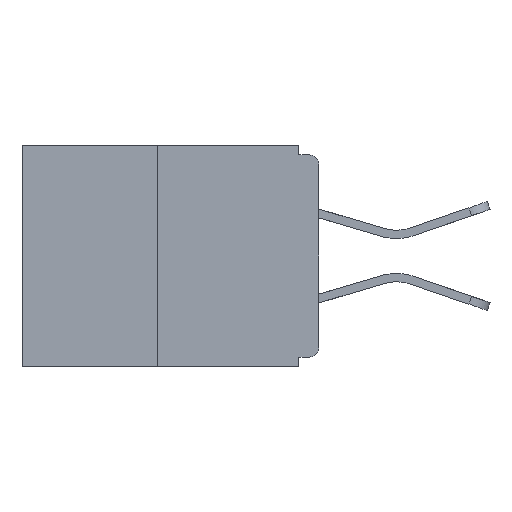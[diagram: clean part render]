
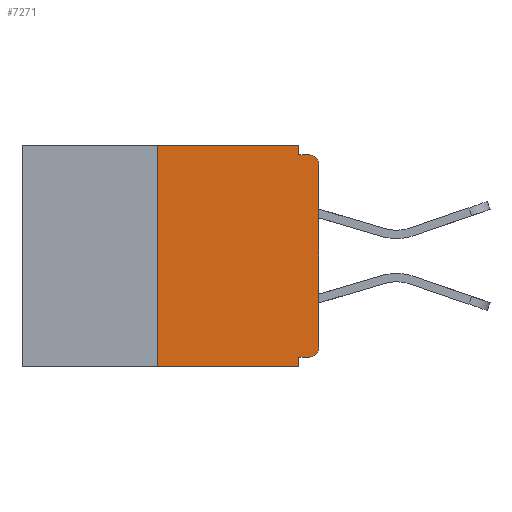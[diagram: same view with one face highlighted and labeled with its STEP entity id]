
A CAD part, left-side view. The second image highlights one B-rep face of the part: STEP entity #7271.
In plain terms, the highlighted planar face has unit normal (-1, 0, 0).
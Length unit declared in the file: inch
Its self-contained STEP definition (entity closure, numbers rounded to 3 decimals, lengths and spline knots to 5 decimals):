
#245 = VECTOR ( 'NONE', #8367, 39.37008 ) ;
#372 = ORIENTED_EDGE ( 'NONE', *, *, #16905, .F. ) ;
#413 = CARTESIAN_POINT ( 'NONE',  ( 0., 0.015, -0.328 ) ) ;
#485 = VECTOR ( 'NONE', #21618, 39.37008 ) ;
#593 = EDGE_CURVE ( 'NONE', #3651, #3572, #9509, .T. ) ;
#948 = EDGE_CURVE ( 'NONE', #8025, #3651, #18871, .T. ) ;
#999 = DIRECTION ( 'NONE',  ( -1., 0., 0. ) ) ;
#1178 = VERTEX_POINT ( 'NONE', #14687 ) ;
#1480 = CARTESIAN_POINT ( 'NONE',  ( 0., 0.25, 0. ) ) ;
#1798 = CARTESIAN_POINT ( 'NONE',  ( 0., 0.031, -0.343 ) ) ;
#1896 = DIRECTION ( 'NONE',  ( 0., 0., -1. ) ) ;
#2040 = CARTESIAN_POINT ( 'NONE',  ( 0., 0.25, -0.343 ) ) ;
#2289 = VECTOR ( 'NONE', #14807, 39.37008 ) ;
#2861 = VERTEX_POINT ( 'NONE', #12835 ) ;
#3013 = VERTEX_POINT ( 'NONE', #2040 ) ;
#3572 = VERTEX_POINT ( 'NONE', #19977 ) ;
#3651 = VERTEX_POINT ( 'NONE', #19838 ) ;
#4171 = DIRECTION ( 'NONE',  ( -1., 0., 0. ) ) ;
#4330 = VERTEX_POINT ( 'NONE', #413 ) ;
#4345 = VECTOR ( 'NONE', #11324, 39.37008 ) ;
#4585 = VERTEX_POINT ( 'NONE', #1798 ) ;
#5065 = CARTESIAN_POINT ( 'NONE',  ( 0., 0.015, -0.015 ) ) ;
#5356 = ORIENTED_EDGE ( 'NONE', *, *, #21210, .T. ) ;
#5528 = CARTESIAN_POINT ( 'NONE',  ( 0., 0.25, 0. ) ) ;
#5738 = CARTESIAN_POINT ( 'NONE',  ( 0., 0.46, -0.343 ) ) ;
#6963 = LINE ( 'NONE', #22767, #2289 ) ;
#7044 = ORIENTED_EDGE ( 'NONE', *, *, #593, .F. ) ;
#7089 = CARTESIAN_POINT ( 'NONE',  ( 0., 0., -0.015 ) ) ;
#7271 = ADVANCED_FACE ( 'NONE', ( #23448 ), #17434, .F. ) ;
#7524 = EDGE_CURVE ( 'NONE', #2861, #7612, #10832, .T. ) ;
#7612 = VERTEX_POINT ( 'NONE', #5065 ) ;
#7782 = DIRECTION ( 'NONE',  ( 1., 0., 0. ) ) ;
#7960 = VECTOR ( 'NONE', #9403, 39.37008 ) ;
#8025 = VERTEX_POINT ( 'NONE', #1480 ) ;
#8233 = ORIENTED_EDGE ( 'NONE', *, *, #20551, .F. ) ;
#8367 = DIRECTION ( 'NONE',  ( 0., 0., -1. ) ) ;
#8378 = CIRCLE ( 'NONE', #24402, 0.015 ) ;
#8411 = EDGE_CURVE ( 'NONE', #3013, #8025, #19294, .T. ) ;
#8814 = DIRECTION ( 'NONE',  ( 0., 0., -1. ) ) ;
#8921 = ORIENTED_EDGE ( 'NONE', *, *, #8411, .F. ) ;
#9403 = DIRECTION ( 'NONE',  ( 0., 0., 1. ) ) ;
#9509 = LINE ( 'NONE', #19525, #23475 ) ;
#9671 = VERTEX_POINT ( 'NONE', #22736 ) ;
#10308 = LINE ( 'NONE', #18119, #245 ) ;
#10349 = DIRECTION ( 'NONE',  ( 0., 1., 0. ) ) ;
#10405 = VECTOR ( 'NONE', #10349, 39.37008 ) ;
#10765 = CARTESIAN_POINT ( 'NONE',  ( 0., 0.015, -0.313 ) ) ;
#10832 = CIRCLE ( 'NONE', #25196, 0.015 ) ;
#11324 = DIRECTION ( 'NONE',  ( 0., -1., 0. ) ) ;
#11654 = CARTESIAN_POINT ( 'NONE',  ( 0., 0.46, 0. ) ) ;
#12570 = ORIENTED_EDGE ( 'NONE', *, *, #14041, .F. ) ;
#12835 = CARTESIAN_POINT ( 'NONE',  ( 0., 0., -0.03 ) ) ;
#14041 = EDGE_CURVE ( 'NONE', #4330, #9671, #14324, .T. ) ;
#14324 = LINE ( 'NONE', #23833, #10405 ) ;
#14687 = CARTESIAN_POINT ( 'NONE',  ( 0., 0., -0.313 ) ) ;
#14807 = DIRECTION ( 'NONE',  ( 0., 0., 1. ) ) ;
#15735 = ORIENTED_EDGE ( 'NONE', *, *, #19790, .T. ) ;
#16737 = LINE ( 'NONE', #7089, #19774 ) ;
#16905 = EDGE_CURVE ( 'NONE', #3572, #7612, #16737, .T. ) ;
#17434 = PLANE ( 'NONE',  #23930 ) ;
#18119 = CARTESIAN_POINT ( 'NONE',  ( 0., 0.031, -0.343 ) ) ;
#18169 = DIRECTION ( 'NONE',  ( 0., 0., -1. ) ) ;
#18871 = LINE ( 'NONE', #24784, #485 ) ;
#18924 = DIRECTION ( 'NONE',  ( 0., -1., 0. ) ) ;
#18945 = EDGE_CURVE ( 'NONE', #1178, #2861, #6963, .T. ) ;
#19294 = LINE ( 'NONE', #5528, #7960 ) ;
#19525 = CARTESIAN_POINT ( 'NONE',  ( 0., 0.031, 0. ) ) ;
#19774 = VECTOR ( 'NONE', #18924, 39.37008 ) ;
#19790 = EDGE_CURVE ( 'NONE', #4330, #1178, #8378, .T. ) ;
#19838 = CARTESIAN_POINT ( 'NONE',  ( 0., 0.031, 0. ) ) ;
#19977 = CARTESIAN_POINT ( 'NONE',  ( 0., 0.031, -0.015 ) ) ;
#20197 = ORIENTED_EDGE ( 'NONE', *, *, #948, .F. ) ;
#20442 = EDGE_LOOP ( 'NONE', ( #20197, #8921, #5356, #8233, #12570, #15735, #23000, #21418, #372, #7044 ) ) ;
#20551 = EDGE_CURVE ( 'NONE', #9671, #4585, #10308, .T. ) ;
#21210 = EDGE_CURVE ( 'NONE', #3013, #4585, #25176, .T. ) ;
#21418 = ORIENTED_EDGE ( 'NONE', *, *, #7524, .T. ) ;
#21618 = DIRECTION ( 'NONE',  ( 0., -1., 0. ) ) ;
#22736 = CARTESIAN_POINT ( 'NONE',  ( 0., 0.031, -0.328 ) ) ;
#22767 = CARTESIAN_POINT ( 'NONE',  ( 0., 0., 0. ) ) ;
#23000 = ORIENTED_EDGE ( 'NONE', *, *, #18945, .T. ) ;
#23448 = FACE_OUTER_BOUND ( 'NONE', #20442, .T. ) ;
#23475 = VECTOR ( 'NONE', #25327, 39.37008 ) ;
#23833 = CARTESIAN_POINT ( 'NONE',  ( 0., 0., -0.328 ) ) ;
#23930 = AXIS2_PLACEMENT_3D ( 'NONE', #11654, #7782, #1896 ) ;
#23972 = CARTESIAN_POINT ( 'NONE',  ( 0., 0.015, -0.03 ) ) ;
#24402 = AXIS2_PLACEMENT_3D ( 'NONE', #10765, #999, #8814 ) ;
#24784 = CARTESIAN_POINT ( 'NONE',  ( 0., 0.46, 0. ) ) ;
#25176 = LINE ( 'NONE', #5738, #4345 ) ;
#25196 = AXIS2_PLACEMENT_3D ( 'NONE', #23972, #4171, #18169 ) ;
#25327 = DIRECTION ( 'NONE',  ( 0., 0., -1. ) ) ;
